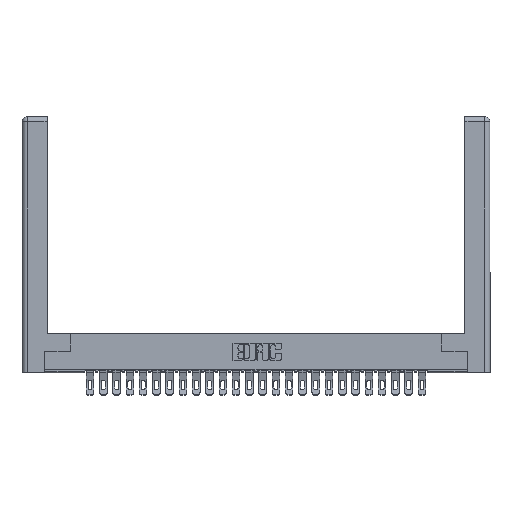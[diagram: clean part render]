
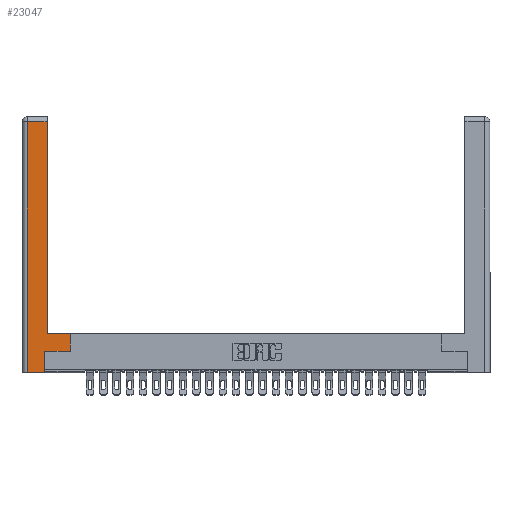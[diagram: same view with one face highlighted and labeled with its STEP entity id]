
A CAD part, top view. The second image highlights one B-rep face of the part: STEP entity #23047.
In plain terms, the highlighted planar face has unit normal (0, 0, 1).
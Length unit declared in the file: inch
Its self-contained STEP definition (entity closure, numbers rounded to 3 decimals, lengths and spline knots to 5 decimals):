
#293 = DIRECTION ( 'NONE',  ( 0., 1., 0. ) ) ;
#714 = CARTESIAN_POINT ( 'NONE',  ( 0., 0., 0. ) ) ;
#1807 = VERTEX_POINT ( 'NONE', #19714 ) ;
#1836 = ORIENTED_EDGE ( 'NONE', *, *, #14642, .T. ) ;
#1947 = VERTEX_POINT ( 'NONE', #30011 ) ;
#2520 = DIRECTION ( 'NONE',  ( 0., 1., 0. ) ) ;
#4404 = LINE ( 'NONE', #16812, #4835 ) ;
#4814 = ORIENTED_EDGE ( 'NONE', *, *, #22803, .T. ) ;
#4835 = VECTOR ( 'NONE', #11526, 39.37008 ) ;
#5586 = LINE ( 'NONE', #7346, #10022 ) ;
#6065 = VERTEX_POINT ( 'NONE', #29537 ) ;
#6104 = PLANE ( 'NONE',  #13678 ) ;
#7346 = CARTESIAN_POINT ( 'NONE',  ( 0.565, 0.45, 0. ) ) ;
#8014 = VERTEX_POINT ( 'NONE', #28009 ) ;
#8576 = CARTESIAN_POINT ( 'NONE',  ( 0.265, 0., 0. ) ) ;
#9378 = LINE ( 'NONE', #26092, #13018 ) ;
#9532 = DIRECTION ( 'NONE',  ( 1., 0., 0. ) ) ;
#10022 = VECTOR ( 'NONE', #30801, 39.37008 ) ;
#10220 = ORIENTED_EDGE ( 'NONE', *, *, #33227, .T. ) ;
#10225 = VECTOR ( 'NONE', #9532, 39.37008 ) ;
#11526 = DIRECTION ( 'NONE',  ( 0., -1., 0. ) ) ;
#11612 = VERTEX_POINT ( 'NONE', #24657 ) ;
#11902 = ORIENTED_EDGE ( 'NONE', *, *, #13482, .T. ) ;
#13018 = VECTOR ( 'NONE', #2520, 39.37008 ) ;
#13238 = DIRECTION ( 'NONE',  ( -1., 0., 0. ) ) ;
#13482 = EDGE_CURVE ( 'NONE', #20415, #17767, #23692, .T. ) ;
#13678 = AXIS2_PLACEMENT_3D ( 'NONE', #714, #13894, #31572 ) ;
#13894 = DIRECTION ( 'NONE',  ( 0., 0., -1. ) ) ;
#14642 = EDGE_CURVE ( 'NONE', #11612, #20415, #29605, .T. ) ;
#15128 = EDGE_CURVE ( 'NONE', #1807, #8014, #30380, .T. ) ;
#16008 = DIRECTION ( 'NONE',  ( 1., 0., 0. ) ) ;
#16321 = CARTESIAN_POINT ( 'NONE',  ( 0.265, 0., 0. ) ) ;
#16675 = LINE ( 'NONE', #8576, #31583 ) ;
#16812 = CARTESIAN_POINT ( 'NONE',  ( 0.0615, 0., 0. ) ) ;
#17210 = DIRECTION ( 'NONE',  ( -1., 0., 0. ) ) ;
#17286 = VERTEX_POINT ( 'NONE', #16321 ) ;
#17767 = VERTEX_POINT ( 'NONE', #28695 ) ;
#19292 = ORIENTED_EDGE ( 'NONE', *, *, #29353, .T. ) ;
#19714 = CARTESIAN_POINT ( 'NONE',  ( 0.265, 0.245, 0. ) ) ;
#20011 = CARTESIAN_POINT ( 'NONE',  ( 0.295, 3., 0. ) ) ;
#20150 = ORIENTED_EDGE ( 'NONE', *, *, #15128, .T. ) ;
#20415 = VERTEX_POINT ( 'NONE', #25181 ) ;
#21725 = VECTOR ( 'NONE', #13238, 39.37008 ) ;
#22803 = EDGE_CURVE ( 'NONE', #8014, #11612, #5586, .T. ) ;
#23047 = ADVANCED_FACE ( 'NONE', ( #32970 ), #6104, .F. ) ;
#23692 = LINE ( 'NONE', #20011, #30111 ) ;
#24657 = CARTESIAN_POINT ( 'NONE',  ( 0.565, 0.45, 0. ) ) ;
#24924 = CARTESIAN_POINT ( 'NONE',  ( 0.295, 0.45, 0. ) ) ;
#25181 = CARTESIAN_POINT ( 'NONE',  ( 0.295, 0.45, 0. ) ) ;
#25602 = VECTOR ( 'NONE', #17210, 39.37008 ) ;
#26092 = CARTESIAN_POINT ( 'NONE',  ( 0.265, 0.245, 0. ) ) ;
#26127 = CARTESIAN_POINT ( 'NONE',  ( 0.0615, 2.94, 0. ) ) ;
#27236 = CARTESIAN_POINT ( 'NONE',  ( 0.565, 0.245, 0. ) ) ;
#28009 = CARTESIAN_POINT ( 'NONE',  ( 0.565, 0.245, 0. ) ) ;
#28695 = CARTESIAN_POINT ( 'NONE',  ( 0.295, 2.94, 0. ) ) ;
#29353 = EDGE_CURVE ( 'NONE', #6065, #17286, #16675, .T. ) ;
#29443 = EDGE_LOOP ( 'NONE', ( #11902, #10220, #29525, #19292, #31650, #20150, #4814, #1836 ) ) ;
#29525 = ORIENTED_EDGE ( 'NONE', *, *, #32273, .T. ) ;
#29537 = CARTESIAN_POINT ( 'NONE',  ( 0.0615, 0., 0. ) ) ;
#29605 = LINE ( 'NONE', #24924, #25602 ) ;
#30011 = CARTESIAN_POINT ( 'NONE',  ( 0.0615, 2.94, 0. ) ) ;
#30111 = VECTOR ( 'NONE', #293, 39.37008 ) ;
#30380 = LINE ( 'NONE', #27236, #10225 ) ;
#30564 = LINE ( 'NONE', #26127, #21725 ) ;
#30732 = EDGE_CURVE ( 'NONE', #17286, #1807, #9378, .T. ) ;
#30801 = DIRECTION ( 'NONE',  ( 0., 1., 0. ) ) ;
#31572 = DIRECTION ( 'NONE',  ( -1., 0., 0. ) ) ;
#31583 = VECTOR ( 'NONE', #16008, 39.37008 ) ;
#31650 = ORIENTED_EDGE ( 'NONE', *, *, #30732, .T. ) ;
#32273 = EDGE_CURVE ( 'NONE', #1947, #6065, #4404, .T. ) ;
#32970 = FACE_OUTER_BOUND ( 'NONE', #29443, .T. ) ;
#33227 = EDGE_CURVE ( 'NONE', #17767, #1947, #30564, .T. ) ;
